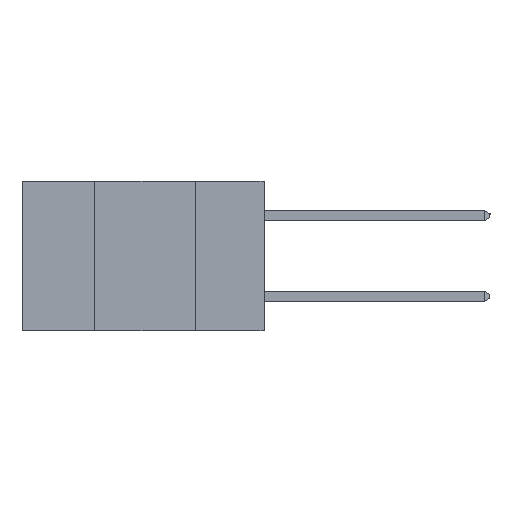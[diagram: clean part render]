
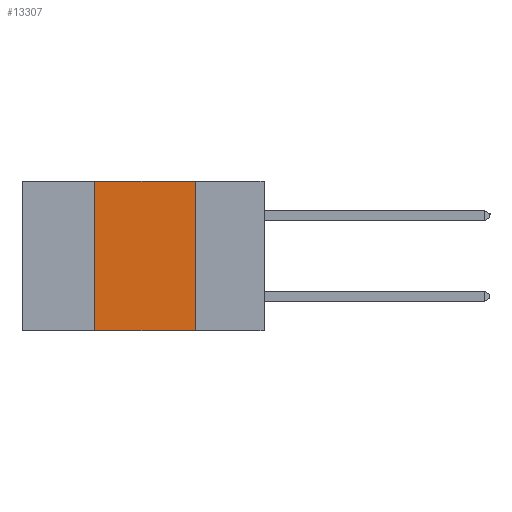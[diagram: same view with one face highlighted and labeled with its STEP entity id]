
A CAD part, left-side view. The second image highlights one B-rep face of the part: STEP entity #13307.
In plain terms, the highlighted planar face has unit normal (-1, 0, 0).
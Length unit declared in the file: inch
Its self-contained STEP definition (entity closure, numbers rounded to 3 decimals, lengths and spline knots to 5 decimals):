
#2190 = LINE ( 'NONE', #18150, #20235 ) ;
#2976 = DIRECTION ( 'NONE',  ( 0., 0., -1. ) ) ;
#2983 = CARTESIAN_POINT ( 'NONE',  ( 0., 0.42, -0.37 ) ) ;
#3424 = AXIS2_PLACEMENT_3D ( 'NONE', #5026, #23177, #23431 ) ;
#5026 = CARTESIAN_POINT ( 'NONE',  ( 0., 0.6, 0. ) ) ;
#5839 = CARTESIAN_POINT ( 'NONE',  ( 0., 0.17, -0.37 ) ) ;
#6187 = VERTEX_POINT ( 'NONE', #5839 ) ;
#6247 = CARTESIAN_POINT ( 'NONE',  ( 0., 0.42, 0. ) ) ;
#7271 = EDGE_CURVE ( 'NONE', #20763, #23099, #22844, .T. ) ;
#7943 = ORIENTED_EDGE ( 'NONE', *, *, #7271, .F. ) ;
#7998 = ORIENTED_EDGE ( 'NONE', *, *, #25510, .T. ) ;
#9142 = DIRECTION ( 'NONE',  ( 0., 0., 1. ) ) ;
#10577 = VERTEX_POINT ( 'NONE', #19107 ) ;
#10869 = ORIENTED_EDGE ( 'NONE', *, *, #13091, .F. ) ;
#11756 = VECTOR ( 'NONE', #19657, 39.37008 ) ;
#11849 = LINE ( 'NONE', #21751, #11756 ) ;
#11968 = VECTOR ( 'NONE', #21797, 39.37008 ) ;
#13091 = EDGE_CURVE ( 'NONE', #23099, #10577, #11849, .T. ) ;
#13307 = ADVANCED_FACE ( 'NONE', ( #14711 ), #15479, .F. ) ;
#14711 = FACE_OUTER_BOUND ( 'NONE', #15717, .T. ) ;
#15414 = CARTESIAN_POINT ( 'NONE',  ( 0., 0.42, -0.37 ) ) ;
#15479 = PLANE ( 'NONE',  #3424 ) ;
#15717 = EDGE_LOOP ( 'NONE', ( #18750, #10869, #7943, #7998 ) ) ;
#17519 = CARTESIAN_POINT ( 'NONE',  ( 0., 0.6, -0.37 ) ) ;
#18150 = CARTESIAN_POINT ( 'NONE',  ( 0., 0.17, -0.37 ) ) ;
#18750 = ORIENTED_EDGE ( 'NONE', *, *, #24363, .F. ) ;
#19107 = CARTESIAN_POINT ( 'NONE',  ( 0., 0.17, 0. ) ) ;
#19657 = DIRECTION ( 'NONE',  ( 0., -1., 0. ) ) ;
#20235 = VECTOR ( 'NONE', #2976, 39.37008 ) ;
#20763 = VERTEX_POINT ( 'NONE', #15414 ) ;
#21423 = LINE ( 'NONE', #17519, #11968 ) ;
#21751 = CARTESIAN_POINT ( 'NONE',  ( 0., 0.6, 0. ) ) ;
#21797 = DIRECTION ( 'NONE',  ( 0., -1., 0. ) ) ;
#21839 = VECTOR ( 'NONE', #9142, 39.37008 ) ;
#22844 = LINE ( 'NONE', #2983, #21839 ) ;
#23099 = VERTEX_POINT ( 'NONE', #6247 ) ;
#23177 = DIRECTION ( 'NONE',  ( 1., 0., 0. ) ) ;
#23431 = DIRECTION ( 'NONE',  ( 0., 0., -1. ) ) ;
#24363 = EDGE_CURVE ( 'NONE', #10577, #6187, #2190, .T. ) ;
#25510 = EDGE_CURVE ( 'NONE', #20763, #6187, #21423, .T. ) ;
